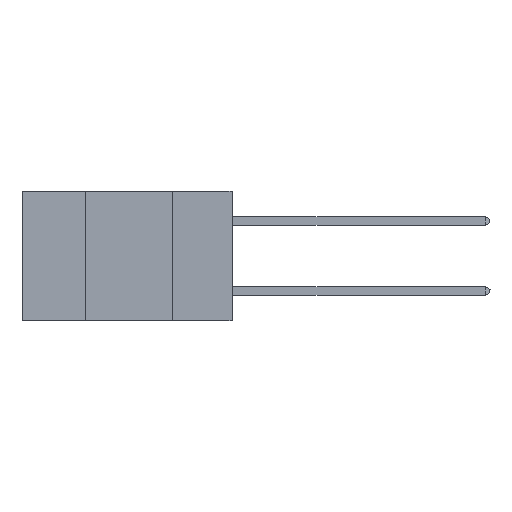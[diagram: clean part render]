
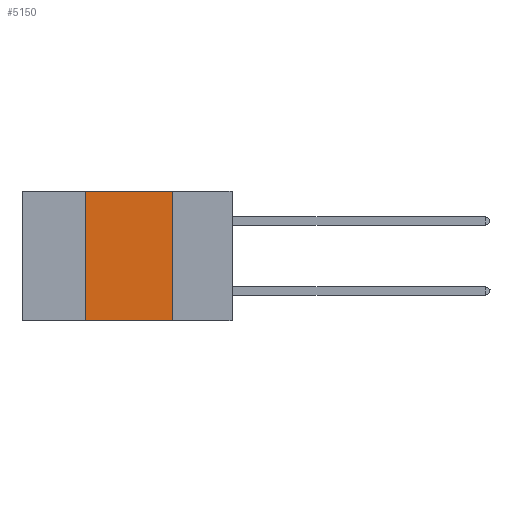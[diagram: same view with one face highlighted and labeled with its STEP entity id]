
A CAD part, left-side view. The second image highlights one B-rep face of the part: STEP entity #5150.
In plain terms, the highlighted planar face has unit normal (-1, 0, 0).
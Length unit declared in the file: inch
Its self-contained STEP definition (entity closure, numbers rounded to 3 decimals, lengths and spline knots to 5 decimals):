
#879 = DIRECTION ( 'NONE',  ( 1., 0., 0. ) ) ;
#1328 = VECTOR ( 'NONE', #2078, 39.37008 ) ;
#2046 = PLANE ( 'NONE',  #5070 ) ;
#2078 = DIRECTION ( 'NONE',  ( 0., 0., 1. ) ) ;
#2965 = CARTESIAN_POINT ( 'NONE',  ( 0., 0.6, 0. ) ) ;
#3883 = CARTESIAN_POINT ( 'NONE',  ( 0., 0.6, 0. ) ) ;
#4323 = ORIENTED_EDGE ( 'NONE', *, *, #16074, .F. ) ;
#4455 = LINE ( 'NONE', #18448, #6192 ) ;
#4642 = VERTEX_POINT ( 'NONE', #18975 ) ;
#5047 = LINE ( 'NONE', #2965, #23002 ) ;
#5070 = AXIS2_PLACEMENT_3D ( 'NONE', #3883, #879, #16840 ) ;
#5150 = ADVANCED_FACE ( 'NONE', ( #23653 ), #2046, .F. ) ;
#5305 = CARTESIAN_POINT ( 'NONE',  ( 0., 0.42, 0. ) ) ;
#6192 = VECTOR ( 'NONE', #13111, 39.37008 ) ;
#6292 = CARTESIAN_POINT ( 'NONE',  ( 0., 0.17, -0.37 ) ) ;
#6510 = EDGE_LOOP ( 'NONE', ( #4323, #9471, #19899, #17280 ) ) ;
#8323 = VERTEX_POINT ( 'NONE', #18143 ) ;
#9471 = ORIENTED_EDGE ( 'NONE', *, *, #18399, .F. ) ;
#10494 = DIRECTION ( 'NONE',  ( 0., 0., -1. ) ) ;
#11144 = LINE ( 'NONE', #5305, #1328 ) ;
#12148 = EDGE_CURVE ( 'NONE', #8323, #23557, #4455, .T. ) ;
#12290 = EDGE_CURVE ( 'NONE', #8323, #4642, #11144, .T. ) ;
#13090 = CARTESIAN_POINT ( 'NONE',  ( 0., 0.17, 0. ) ) ;
#13111 = DIRECTION ( 'NONE',  ( 0., -1., 0. ) ) ;
#14535 = CARTESIAN_POINT ( 'NONE',  ( 0., 0.17, 0. ) ) ;
#16074 = EDGE_CURVE ( 'NONE', #18884, #23557, #17649, .T. ) ;
#16840 = DIRECTION ( 'NONE',  ( 0., 0., -1. ) ) ;
#17280 = ORIENTED_EDGE ( 'NONE', *, *, #12148, .T. ) ;
#17649 = LINE ( 'NONE', #14535, #21737 ) ;
#18143 = CARTESIAN_POINT ( 'NONE',  ( 0., 0.42, -0.37 ) ) ;
#18399 = EDGE_CURVE ( 'NONE', #4642, #18884, #5047, .T. ) ;
#18448 = CARTESIAN_POINT ( 'NONE',  ( 0., 0.6, -0.37 ) ) ;
#18884 = VERTEX_POINT ( 'NONE', #13090 ) ;
#18975 = CARTESIAN_POINT ( 'NONE',  ( 0., 0.42, 0. ) ) ;
#19899 = ORIENTED_EDGE ( 'NONE', *, *, #12290, .F. ) ;
#21737 = VECTOR ( 'NONE', #10494, 39.37008 ) ;
#23002 = VECTOR ( 'NONE', #23584, 39.37008 ) ;
#23557 = VERTEX_POINT ( 'NONE', #6292 ) ;
#23584 = DIRECTION ( 'NONE',  ( 0., -1., 0. ) ) ;
#23653 = FACE_OUTER_BOUND ( 'NONE', #6510, .T. ) ;
